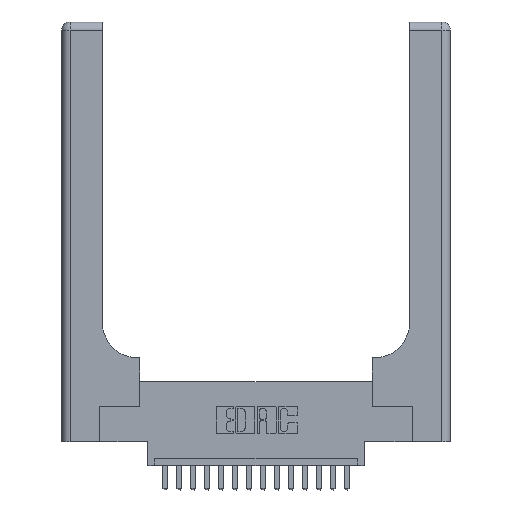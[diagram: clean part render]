
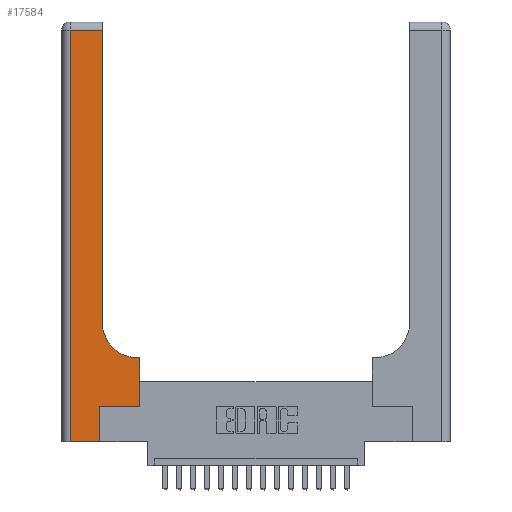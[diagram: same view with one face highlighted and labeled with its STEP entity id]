
A CAD part, top view. The second image highlights one B-rep face of the part: STEP entity #17584.
In plain terms, the highlighted planar face has unit normal (0, 0, 1).
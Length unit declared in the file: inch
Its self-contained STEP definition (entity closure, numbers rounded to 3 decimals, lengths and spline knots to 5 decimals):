
#62 = ORIENTED_EDGE ( 'NONE', *, *, #11247, .T. ) ;
#609 = LINE ( 'NONE', #17558, #6277 ) ;
#708 = CIRCLE ( 'NONE', #17267, 0.25 ) ;
#1001 = PLANE ( 'NONE',  #11091 ) ;
#1354 = LINE ( 'NONE', #4929, #11371 ) ;
#2093 = VECTOR ( 'NONE', #11570, 39.37008 ) ;
#2208 = CARTESIAN_POINT ( 'NONE',  ( 0.06, 2.94, 0.37 ) ) ;
#2539 = EDGE_CURVE ( 'NONE', #2694, #5560, #708, .T. ) ;
#2620 = DIRECTION ( 'NONE',  ( 0., 0., -1. ) ) ;
#2694 = VERTEX_POINT ( 'NONE', #13571 ) ;
#2853 = LINE ( 'NONE', #17438, #12853 ) ;
#2870 = ORIENTED_EDGE ( 'NONE', *, *, #6612, .T. ) ;
#3232 = LINE ( 'NONE', #18791, #15171 ) ;
#3297 = DIRECTION ( 'NONE',  ( -1., 0., 0. ) ) ;
#3309 = VECTOR ( 'NONE', #12570, 39.37008 ) ;
#3835 = VERTEX_POINT ( 'NONE', #15710 ) ;
#3895 = DIRECTION ( 'NONE',  ( 0., 1., 0. ) ) ;
#3923 = CARTESIAN_POINT ( 'NONE',  ( 0.5415, 0.85, 0.37 ) ) ;
#3985 = FACE_OUTER_BOUND ( 'NONE', #11024, .T. ) ;
#4433 = CARTESIAN_POINT ( 'NONE',  ( 0.2915, 0.85, 0.37 ) ) ;
#4744 = CARTESIAN_POINT ( 'NONE',  ( 0.269, 0.25, 0.37 ) ) ;
#4929 = CARTESIAN_POINT ( 'NONE',  ( 0., 2.94, 0.37 ) ) ;
#5491 = DIRECTION ( 'NONE',  ( 1., 0., 0. ) ) ;
#5560 = VERTEX_POINT ( 'NONE', #4433 ) ;
#5618 = DIRECTION ( 'NONE',  ( -1., 0., 0. ) ) ;
#5641 = LINE ( 'NONE', #15787, #3309 ) ;
#6205 = EDGE_CURVE ( 'NONE', #3835, #7940, #1354, .T. ) ;
#6277 = VECTOR ( 'NONE', #11652, 39.37008 ) ;
#6612 = EDGE_CURVE ( 'NONE', #7940, #18737, #3232, .T. ) ;
#7643 = VERTEX_POINT ( 'NONE', #16457 ) ;
#7732 = VERTEX_POINT ( 'NONE', #16999 ) ;
#7940 = VERTEX_POINT ( 'NONE', #2208 ) ;
#8256 = DIRECTION ( 'NONE',  ( 0., 1., 0. ) ) ;
#8643 = ORIENTED_EDGE ( 'NONE', *, *, #12089, .T. ) ;
#9026 = CARTESIAN_POINT ( 'NONE',  ( 0.269, 0., 0.37 ) ) ;
#9303 = ORIENTED_EDGE ( 'NONE', *, *, #2539, .T. ) ;
#9470 = VERTEX_POINT ( 'NONE', #9026 ) ;
#9600 = DIRECTION ( 'NONE',  ( 0., -1., 0. ) ) ;
#10226 = ORIENTED_EDGE ( 'NONE', *, *, #6205, .T. ) ;
#10524 = EDGE_CURVE ( 'NONE', #9470, #13228, #15967, .T. ) ;
#10792 = EDGE_CURVE ( 'NONE', #7732, #7643, #2853, .T. ) ;
#11024 = EDGE_LOOP ( 'NONE', ( #62, #10226, #2870, #14189, #17528, #15345, #16666, #8643, #9303 ) ) ;
#11091 = AXIS2_PLACEMENT_3D ( 'NONE', #16582, #2620, #5618 ) ;
#11153 = VECTOR ( 'NONE', #3895, 39.37008 ) ;
#11247 = EDGE_CURVE ( 'NONE', #5560, #3835, #5641, .T. ) ;
#11371 = VECTOR ( 'NONE', #3297, 39.37008 ) ;
#11570 = DIRECTION ( 'NONE',  ( 1., 0., 0. ) ) ;
#11652 = DIRECTION ( 'NONE',  ( 1., 0., 0. ) ) ;
#12089 = EDGE_CURVE ( 'NONE', #7643, #2694, #18818, .T. ) ;
#12570 = DIRECTION ( 'NONE',  ( 0., 1., 0. ) ) ;
#12853 = VECTOR ( 'NONE', #8256, 39.37008 ) ;
#12979 = EDGE_CURVE ( 'NONE', #13228, #7732, #19003, .T. ) ;
#13228 = VERTEX_POINT ( 'NONE', #4744 ) ;
#13571 = CARTESIAN_POINT ( 'NONE',  ( 0.5415, 0.6, 0.37 ) ) ;
#14189 = ORIENTED_EDGE ( 'NONE', *, *, #14196, .T. ) ;
#14196 = EDGE_CURVE ( 'NONE', #18737, #9470, #609, .T. ) ;
#14671 = DIRECTION ( 'NONE',  ( 0., 0., -1. ) ) ;
#14834 = CARTESIAN_POINT ( 'NONE',  ( 0.06, 0., 0.37 ) ) ;
#15171 = VECTOR ( 'NONE', #9600, 39.37008 ) ;
#15345 = ORIENTED_EDGE ( 'NONE', *, *, #12979, .T. ) ;
#15710 = CARTESIAN_POINT ( 'NONE',  ( 0.2915, 2.94, 0.37 ) ) ;
#15787 = CARTESIAN_POINT ( 'NONE',  ( 0.2915, 3., 0.37 ) ) ;
#15967 = LINE ( 'NONE', #19425, #11153 ) ;
#16457 = CARTESIAN_POINT ( 'NONE',  ( 0.5585, 0.6, 0.37 ) ) ;
#16582 = CARTESIAN_POINT ( 'NONE',  ( 0., 3., 0.37 ) ) ;
#16666 = ORIENTED_EDGE ( 'NONE', *, *, #10792, .T. ) ;
#16999 = CARTESIAN_POINT ( 'NONE',  ( 0.5585, 0.25, 0.37 ) ) ;
#17267 = AXIS2_PLACEMENT_3D ( 'NONE', #3923, #14671, #5491 ) ;
#17429 = DIRECTION ( 'NONE',  ( -1., 0., 0. ) ) ;
#17438 = CARTESIAN_POINT ( 'NONE',  ( 0.5585, 0.25, 0.37 ) ) ;
#17528 = ORIENTED_EDGE ( 'NONE', *, *, #10524, .T. ) ;
#17558 = CARTESIAN_POINT ( 'NONE',  ( 0., 0., 0.37 ) ) ;
#17584 = ADVANCED_FACE ( 'NONE', ( #3985 ), #1001, .F. ) ;
#17829 = VECTOR ( 'NONE', #17429, 39.37008 ) ;
#18737 = VERTEX_POINT ( 'NONE', #14834 ) ;
#18767 = CARTESIAN_POINT ( 'NONE',  ( 0.2915, 0.6, 0.37 ) ) ;
#18791 = CARTESIAN_POINT ( 'NONE',  ( 0.06, 3., 0.37 ) ) ;
#18818 = LINE ( 'NONE', #18767, #17829 ) ;
#19003 = LINE ( 'NONE', #19368, #2093 ) ;
#19368 = CARTESIAN_POINT ( 'NONE',  ( 0.269, 0.25, 0.37 ) ) ;
#19425 = CARTESIAN_POINT ( 'NONE',  ( 0.269, 0., 0.37 ) ) ;
